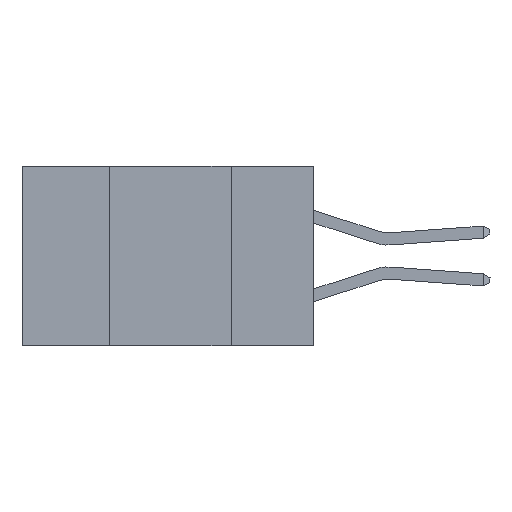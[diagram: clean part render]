
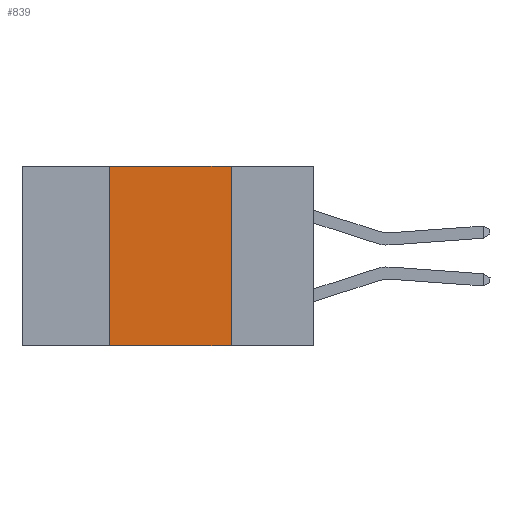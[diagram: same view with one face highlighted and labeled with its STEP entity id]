
A CAD part, left-side view. The second image highlights one B-rep face of the part: STEP entity #839.
In plain terms, the highlighted planar face has unit normal (-1, 0, 0).
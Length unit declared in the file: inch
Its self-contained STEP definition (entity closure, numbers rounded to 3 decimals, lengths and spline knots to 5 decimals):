
#658 = CARTESIAN_POINT ( 'NONE',  ( 0., 0.6, 0. ) ) ;
#698 = DIRECTION ( 'NONE',  ( 0., 0., -1. ) ) ;
#839 = ADVANCED_FACE ( 'NONE', ( #10041 ), #6115, .F. ) ;
#857 = LINE ( 'NONE', #7277, #10373 ) ;
#902 = CARTESIAN_POINT ( 'NONE',  ( 0., 0.17, 0. ) ) ;
#1764 = AXIS2_PLACEMENT_3D ( 'NONE', #658, #9748, #698 ) ;
#2489 = CARTESIAN_POINT ( 'NONE',  ( 0., 0.42, -0.37 ) ) ;
#2621 = VECTOR ( 'NONE', #4976, 39.37008 ) ;
#3180 = EDGE_CURVE ( 'NONE', #10487, #10336, #10961, .T. ) ;
#3338 = DIRECTION ( 'NONE',  ( 0., 0., -1. ) ) ;
#3372 = CARTESIAN_POINT ( 'NONE',  ( 0., 0.17, 0. ) ) ;
#3729 = VECTOR ( 'NONE', #11429, 39.37008 ) ;
#3801 = VERTEX_POINT ( 'NONE', #10932 ) ;
#4350 = VERTEX_POINT ( 'NONE', #2489 ) ;
#4555 = EDGE_CURVE ( 'NONE', #4350, #10487, #857, .T. ) ;
#4976 = DIRECTION ( 'NONE',  ( 0., -1., 0. ) ) ;
#5563 = ORIENTED_EDGE ( 'NONE', *, *, #7886, .F. ) ;
#6115 = PLANE ( 'NONE',  #1764 ) ;
#6563 = ORIENTED_EDGE ( 'NONE', *, *, #3180, .F. ) ;
#7277 = CARTESIAN_POINT ( 'NONE',  ( 0., 0.42, 0. ) ) ;
#7886 = EDGE_CURVE ( 'NONE', #10336, #3801, #11103, .T. ) ;
#8053 = DIRECTION ( 'NONE',  ( 0., 0., 1. ) ) ;
#9148 = EDGE_LOOP ( 'NONE', ( #5563, #6563, #10313, #9619 ) ) ;
#9297 = EDGE_CURVE ( 'NONE', #4350, #3801, #10939, .T. ) ;
#9619 = ORIENTED_EDGE ( 'NONE', *, *, #9297, .T. ) ;
#9748 = DIRECTION ( 'NONE',  ( 1., 0., 0. ) ) ;
#10041 = FACE_OUTER_BOUND ( 'NONE', #9148, .T. ) ;
#10313 = ORIENTED_EDGE ( 'NONE', *, *, #4555, .F. ) ;
#10336 = VERTEX_POINT ( 'NONE', #902 ) ;
#10373 = VECTOR ( 'NONE', #8053, 39.37008 ) ;
#10487 = VERTEX_POINT ( 'NONE', #10627 ) ;
#10512 = CARTESIAN_POINT ( 'NONE',  ( 0., 0.6, 0. ) ) ;
#10627 = CARTESIAN_POINT ( 'NONE',  ( 0., 0.42, 0. ) ) ;
#10724 = CARTESIAN_POINT ( 'NONE',  ( 0., 0.6, -0.37 ) ) ;
#10932 = CARTESIAN_POINT ( 'NONE',  ( 0., 0.17, -0.37 ) ) ;
#10939 = LINE ( 'NONE', #10724, #3729 ) ;
#10961 = LINE ( 'NONE', #10512, #2621 ) ;
#10965 = VECTOR ( 'NONE', #3338, 39.37008 ) ;
#11103 = LINE ( 'NONE', #3372, #10965 ) ;
#11429 = DIRECTION ( 'NONE',  ( 0., -1., 0. ) ) ;
